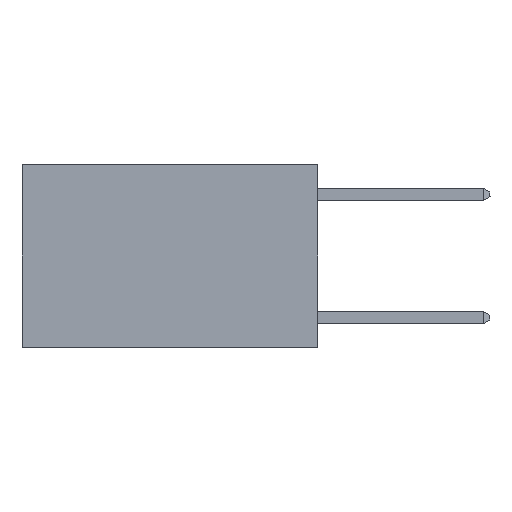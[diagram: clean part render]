
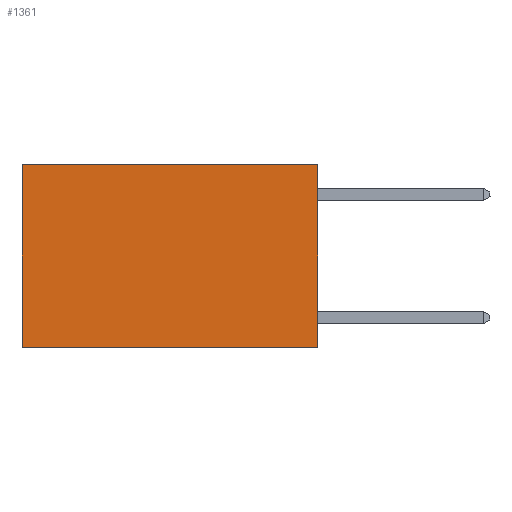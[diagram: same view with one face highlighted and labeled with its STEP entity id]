
A CAD part, left-side view. The second image highlights one B-rep face of the part: STEP entity #1361.
In plain terms, the highlighted planar face has unit normal (-1, 0, 0).
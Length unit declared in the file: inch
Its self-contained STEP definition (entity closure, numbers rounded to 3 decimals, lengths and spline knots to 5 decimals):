
#404 = CARTESIAN_POINT ( 'NONE',  ( 0.2625, 0., 0. ) ) ;
#495 = DIRECTION ( 'NONE',  ( 0., 1., 0. ) ) ;
#1361 = ADVANCED_FACE ( 'NONE', ( #27703 ), #6683, .F. ) ;
#3017 = DIRECTION ( 'NONE',  ( 0., 1., 0. ) ) ;
#4100 = VERTEX_POINT ( 'NONE', #7728 ) ;
#4154 = EDGE_CURVE ( 'NONE', #9873, #15659, #15868, .T. ) ;
#4913 = ORIENTED_EDGE ( 'NONE', *, *, #20512, .T. ) ;
#5146 = CARTESIAN_POINT ( 'NONE',  ( 0.2625, 0.6, 0. ) ) ;
#6683 = PLANE ( 'NONE',  #19944 ) ;
#7125 = DIRECTION ( 'NONE',  ( 0., 0., -1. ) ) ;
#7452 = CARTESIAN_POINT ( 'NONE',  ( 0.2625, 0.6, 0. ) ) ;
#7728 = CARTESIAN_POINT ( 'NONE',  ( 0.2625, 0.6, -0.37 ) ) ;
#8438 = VERTEX_POINT ( 'NONE', #5146 ) ;
#8483 = VECTOR ( 'NONE', #13409, 39.37008 ) ;
#9471 = CARTESIAN_POINT ( 'NONE',  ( 0.2625, 0., -0.37 ) ) ;
#9616 = DIRECTION ( 'NONE',  ( 0., 0., -1. ) ) ;
#9873 = VERTEX_POINT ( 'NONE', #12371 ) ;
#11410 = CARTESIAN_POINT ( 'NONE',  ( 0.2625, 0., 0. ) ) ;
#12371 = CARTESIAN_POINT ( 'NONE',  ( 0.2625, 0., 0. ) ) ;
#13409 = DIRECTION ( 'NONE',  ( 0., 0., -1. ) ) ;
#14306 = CARTESIAN_POINT ( 'NONE',  ( 0.2625, 0., -0.37 ) ) ;
#14408 = ORIENTED_EDGE ( 'NONE', *, *, #16929, .T. ) ;
#15659 = VERTEX_POINT ( 'NONE', #9471 ) ;
#15868 = LINE ( 'NONE', #11410, #8483 ) ;
#16063 = CARTESIAN_POINT ( 'NONE',  ( 0.2625, 0., 0. ) ) ;
#16929 = EDGE_CURVE ( 'NONE', #8438, #4100, #23717, .T. ) ;
#17922 = ORIENTED_EDGE ( 'NONE', *, *, #25285, .F. ) ;
#19944 = AXIS2_PLACEMENT_3D ( 'NONE', #16063, #25395, #7125 ) ;
#20512 = EDGE_CURVE ( 'NONE', #9873, #8438, #21729, .T. ) ;
#21703 = VECTOR ( 'NONE', #495, 39.37008 ) ;
#21729 = LINE ( 'NONE', #404, #22982 ) ;
#22982 = VECTOR ( 'NONE', #3017, 39.37008 ) ;
#23411 = VECTOR ( 'NONE', #9616, 39.37008 ) ;
#23717 = LINE ( 'NONE', #7452, #23411 ) ;
#23818 = EDGE_LOOP ( 'NONE', ( #14408, #17922, #24238, #4913 ) ) ;
#24238 = ORIENTED_EDGE ( 'NONE', *, *, #4154, .F. ) ;
#25285 = EDGE_CURVE ( 'NONE', #15659, #4100, #26241, .T. ) ;
#25395 = DIRECTION ( 'NONE',  ( 1., 0., 0. ) ) ;
#26241 = LINE ( 'NONE', #14306, #21703 ) ;
#27703 = FACE_OUTER_BOUND ( 'NONE', #23818, .T. ) ;
